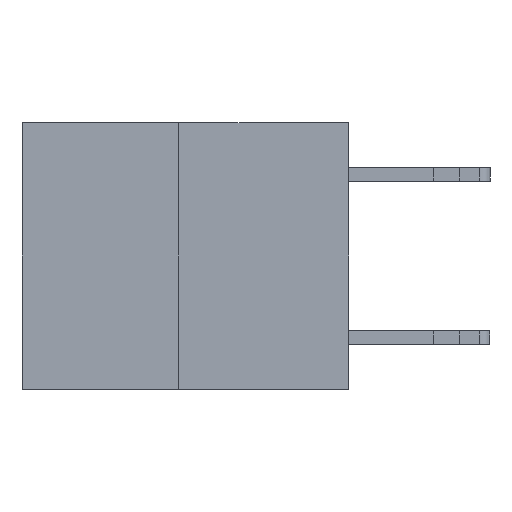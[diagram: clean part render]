
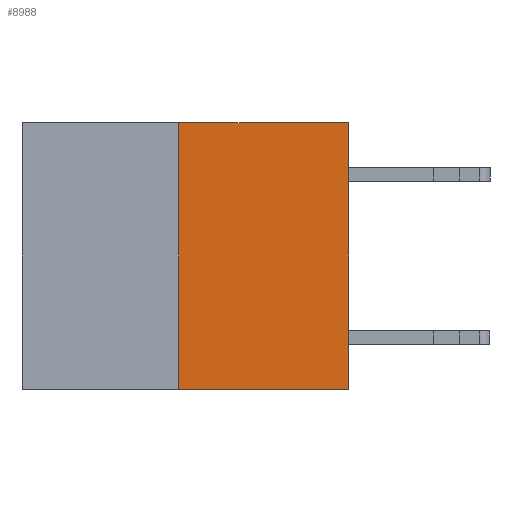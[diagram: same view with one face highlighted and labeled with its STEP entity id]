
A CAD part, left-side view. The second image highlights one B-rep face of the part: STEP entity #8988.
In plain terms, the highlighted planar face has unit normal (-1, 0, 0).
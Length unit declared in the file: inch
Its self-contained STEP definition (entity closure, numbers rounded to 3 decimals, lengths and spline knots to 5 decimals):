
#426 = FACE_OUTER_BOUND ( 'NONE', #9967, .T. ) ;
#783 = LINE ( 'NONE', #4317, #8754 ) ;
#1036 = VERTEX_POINT ( 'NONE', #14833 ) ;
#1159 = AXIS2_PLACEMENT_3D ( 'NONE', #2191, #10460, #11502 ) ;
#1632 = CARTESIAN_POINT ( 'NONE',  ( 0., 0.312, 0. ) ) ;
#1741 = EDGE_CURVE ( 'NONE', #11678, #1036, #11592, .T. ) ;
#2158 = EDGE_CURVE ( 'NONE', #1036, #2384, #15272, .T. ) ;
#2191 = CARTESIAN_POINT ( 'NONE',  ( 0., 0.6, 0. ) ) ;
#2384 = VERTEX_POINT ( 'NONE', #14772 ) ;
#2466 = DIRECTION ( 'NONE',  ( 0., 0., 1. ) ) ;
#2893 = VECTOR ( 'NONE', #7698, 39.37008 ) ;
#3386 = LINE ( 'NONE', #14588, #5798 ) ;
#4317 = CARTESIAN_POINT ( 'NONE',  ( 0., 0.6, 0. ) ) ;
#5624 = EDGE_CURVE ( 'NONE', #11678, #12023, #3386, .T. ) ;
#5798 = VECTOR ( 'NONE', #9943, 39.37008 ) ;
#5848 = ORIENTED_EDGE ( 'NONE', *, *, #5624, .F. ) ;
#7060 = CARTESIAN_POINT ( 'NONE',  ( 0., 0., 0. ) ) ;
#7698 = DIRECTION ( 'NONE',  ( 0., -1., 0. ) ) ;
#8113 = PLANE ( 'NONE',  #1159 ) ;
#8174 = ORIENTED_EDGE ( 'NONE', *, *, #10250, .F. ) ;
#8754 = VECTOR ( 'NONE', #12700, 39.37008 ) ;
#8988 = ADVANCED_FACE ( 'NONE', ( #426 ), #8113, .F. ) ;
#9943 = DIRECTION ( 'NONE',  ( 0., 0., 1. ) ) ;
#9967 = EDGE_LOOP ( 'NONE', ( #5848, #12383, #13661, #8174 ) ) ;
#10250 = EDGE_CURVE ( 'NONE', #12023, #2384, #783, .T. ) ;
#10344 = CARTESIAN_POINT ( 'NONE',  ( 0., 0.312, -0.49 ) ) ;
#10460 = DIRECTION ( 'NONE',  ( 1., 0., 0. ) ) ;
#11297 = CARTESIAN_POINT ( 'NONE',  ( 0., 0.6, -0.49 ) ) ;
#11502 = DIRECTION ( 'NONE',  ( 0., 0., -1. ) ) ;
#11592 = LINE ( 'NONE', #11297, #2893 ) ;
#11678 = VERTEX_POINT ( 'NONE', #10344 ) ;
#12023 = VERTEX_POINT ( 'NONE', #1632 ) ;
#12383 = ORIENTED_EDGE ( 'NONE', *, *, #1741, .T. ) ;
#12700 = DIRECTION ( 'NONE',  ( 0., -1., 0. ) ) ;
#13661 = ORIENTED_EDGE ( 'NONE', *, *, #2158, .T. ) ;
#14588 = CARTESIAN_POINT ( 'NONE',  ( 0., 0.312, -0.49 ) ) ;
#14772 = CARTESIAN_POINT ( 'NONE',  ( 0., 0., 0. ) ) ;
#14833 = CARTESIAN_POINT ( 'NONE',  ( 0., 0., -0.49 ) ) ;
#15097 = VECTOR ( 'NONE', #2466, 39.37008 ) ;
#15272 = LINE ( 'NONE', #7060, #15097 ) ;
